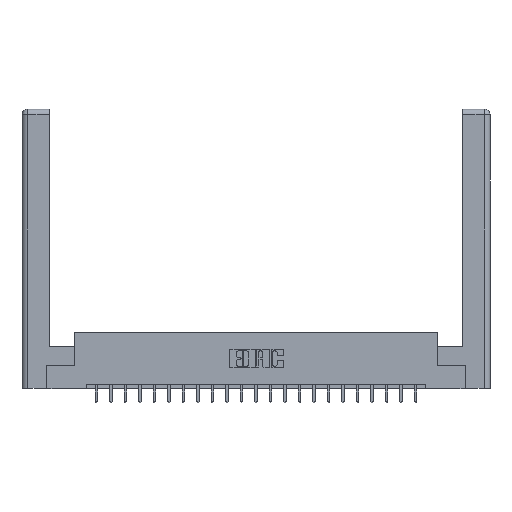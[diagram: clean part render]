
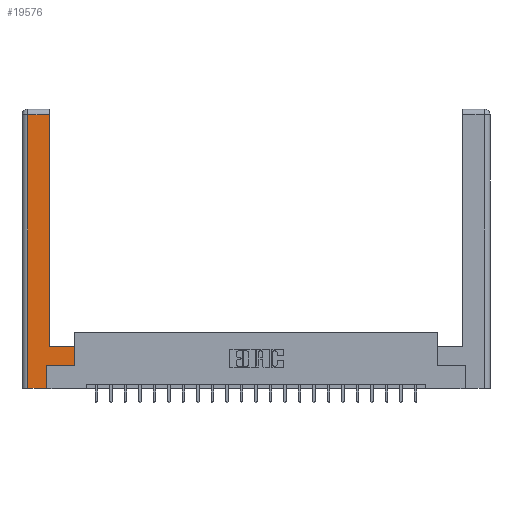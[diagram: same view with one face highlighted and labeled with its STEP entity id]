
A CAD part, top view. The second image highlights one B-rep face of the part: STEP entity #19576.
In plain terms, the highlighted planar face has unit normal (0, 0, 1).
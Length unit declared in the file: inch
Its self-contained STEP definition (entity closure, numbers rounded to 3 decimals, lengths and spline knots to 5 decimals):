
#650 = CARTESIAN_POINT ( 'NONE',  ( 0.265, 0.245, 0. ) ) ;
#871 = VERTEX_POINT ( 'NONE', #13557 ) ;
#963 = CARTESIAN_POINT ( 'NONE',  ( 0.0615, 0., 0. ) ) ;
#1499 = CARTESIAN_POINT ( 'NONE',  ( 0.295, 3., 0. ) ) ;
#1527 = CARTESIAN_POINT ( 'NONE',  ( 0.565, 0.45, 0. ) ) ;
#2704 = ORIENTED_EDGE ( 'NONE', *, *, #18088, .T. ) ;
#3085 = LINE ( 'NONE', #14971, #22797 ) ;
#3601 = VECTOR ( 'NONE', #20083, 39.37008 ) ;
#3816 = VECTOR ( 'NONE', #20524, 39.37008 ) ;
#3907 = EDGE_CURVE ( 'NONE', #6865, #871, #14866, .T. ) ;
#4080 = CARTESIAN_POINT ( 'NONE',  ( 0.265, 0., 0. ) ) ;
#4217 = VECTOR ( 'NONE', #20698, 39.37008 ) ;
#4467 = ORIENTED_EDGE ( 'NONE', *, *, #3907, .T. ) ;
#4871 = AXIS2_PLACEMENT_3D ( 'NONE', #21857, #18380, #18453 ) ;
#5466 = VECTOR ( 'NONE', #8902, 39.37008 ) ;
#5597 = LINE ( 'NONE', #4080, #21410 ) ;
#5888 = LINE ( 'NONE', #10033, #4217 ) ;
#5934 = CARTESIAN_POINT ( 'NONE',  ( 0.265, 0.245, 0. ) ) ;
#6845 = LINE ( 'NONE', #12143, #5466 ) ;
#6865 = VERTEX_POINT ( 'NONE', #19380 ) ;
#7364 = EDGE_CURVE ( 'NONE', #19651, #18896, #5597, .T. ) ;
#7394 = EDGE_CURVE ( 'NONE', #14835, #10254, #3085, .T. ) ;
#8234 = EDGE_CURVE ( 'NONE', #871, #14128, #5888, .T. ) ;
#8817 = VECTOR ( 'NONE', #16620, 39.37008 ) ;
#8836 = CARTESIAN_POINT ( 'NONE',  ( 0.565, 0.245, 0. ) ) ;
#8840 = CARTESIAN_POINT ( 'NONE',  ( 0.565, 0.245, 0. ) ) ;
#8902 = DIRECTION ( 'NONE',  ( -1., 0., 0. ) ) ;
#9393 = ORIENTED_EDGE ( 'NONE', *, *, #8234, .T. ) ;
#9400 = EDGE_LOOP ( 'NONE', ( #4467, #9393, #20188, #14327, #2704, #13483, #12579, #11542 ) ) ;
#10024 = EDGE_CURVE ( 'NONE', #19062, #14835, #14917, .T. ) ;
#10033 = CARTESIAN_POINT ( 'NONE',  ( 0.0615, 2.94, 0. ) ) ;
#10254 = VERTEX_POINT ( 'NONE', #1527 ) ;
#10872 = DIRECTION ( 'NONE',  ( 1., 0., 0. ) ) ;
#11536 = DIRECTION ( 'NONE',  ( 0., 1., 0. ) ) ;
#11542 = ORIENTED_EDGE ( 'NONE', *, *, #11626, .T. ) ;
#11626 = EDGE_CURVE ( 'NONE', #10254, #6865, #6845, .T. ) ;
#12143 = CARTESIAN_POINT ( 'NONE',  ( 0.295, 0.45, 0. ) ) ;
#12579 = ORIENTED_EDGE ( 'NONE', *, *, #7394, .T. ) ;
#13483 = ORIENTED_EDGE ( 'NONE', *, *, #10024, .T. ) ;
#13557 = CARTESIAN_POINT ( 'NONE',  ( 0.295, 2.94, 0. ) ) ;
#13807 = CARTESIAN_POINT ( 'NONE',  ( 0.265, 0., 0. ) ) ;
#14000 = CARTESIAN_POINT ( 'NONE',  ( 0.0615, 0., 0. ) ) ;
#14128 = VERTEX_POINT ( 'NONE', #21485 ) ;
#14327 = ORIENTED_EDGE ( 'NONE', *, *, #7364, .T. ) ;
#14835 = VERTEX_POINT ( 'NONE', #8840 ) ;
#14866 = LINE ( 'NONE', #1499, #18486 ) ;
#14917 = LINE ( 'NONE', #8836, #3601 ) ;
#14971 = CARTESIAN_POINT ( 'NONE',  ( 0.565, 0.45, 0. ) ) ;
#15472 = LINE ( 'NONE', #650, #8817 ) ;
#15852 = DIRECTION ( 'NONE',  ( 0., 1., 0. ) ) ;
#16620 = DIRECTION ( 'NONE',  ( 0., 1., 0. ) ) ;
#18088 = EDGE_CURVE ( 'NONE', #18896, #19062, #15472, .T. ) ;
#18380 = DIRECTION ( 'NONE',  ( 0., 0., -1. ) ) ;
#18453 = DIRECTION ( 'NONE',  ( -1., 0., 0. ) ) ;
#18486 = VECTOR ( 'NONE', #15852, 39.37008 ) ;
#18789 = EDGE_CURVE ( 'NONE', #14128, #19651, #22091, .T. ) ;
#18896 = VERTEX_POINT ( 'NONE', #13807 ) ;
#19062 = VERTEX_POINT ( 'NONE', #5934 ) ;
#19380 = CARTESIAN_POINT ( 'NONE',  ( 0.295, 0.45, 0. ) ) ;
#19576 = ADVANCED_FACE ( 'NONE', ( #22626 ), #21782, .F. ) ;
#19651 = VERTEX_POINT ( 'NONE', #14000 ) ;
#20083 = DIRECTION ( 'NONE',  ( 1., 0., 0. ) ) ;
#20188 = ORIENTED_EDGE ( 'NONE', *, *, #18789, .T. ) ;
#20524 = DIRECTION ( 'NONE',  ( 0., -1., 0. ) ) ;
#20698 = DIRECTION ( 'NONE',  ( -1., 0., 0. ) ) ;
#21410 = VECTOR ( 'NONE', #10872, 39.37008 ) ;
#21485 = CARTESIAN_POINT ( 'NONE',  ( 0.0615, 2.94, 0. ) ) ;
#21782 = PLANE ( 'NONE',  #4871 ) ;
#21857 = CARTESIAN_POINT ( 'NONE',  ( 0., 0., 0. ) ) ;
#22091 = LINE ( 'NONE', #963, #3816 ) ;
#22626 = FACE_OUTER_BOUND ( 'NONE', #9400, .T. ) ;
#22797 = VECTOR ( 'NONE', #11536, 39.37008 ) ;
